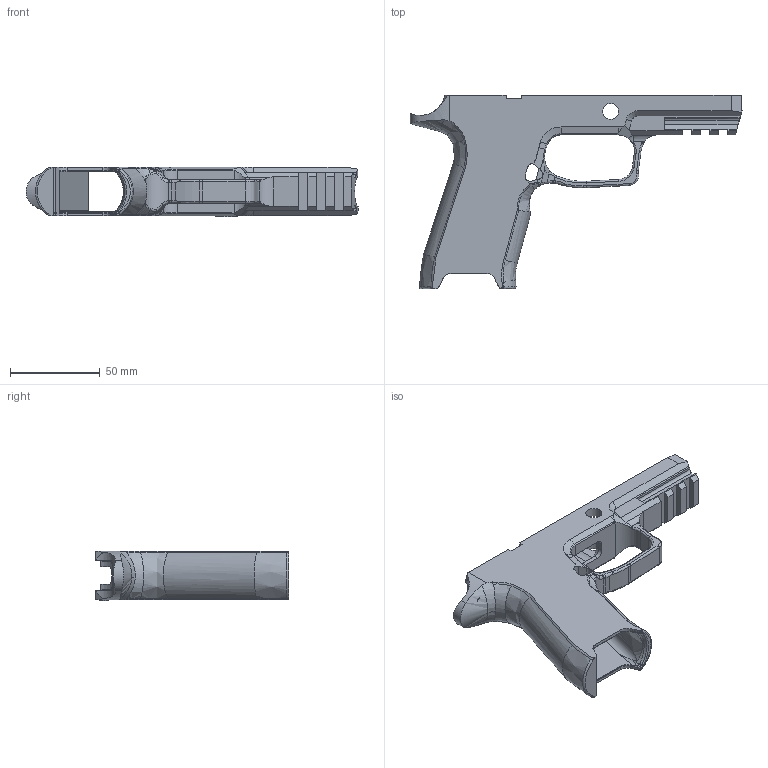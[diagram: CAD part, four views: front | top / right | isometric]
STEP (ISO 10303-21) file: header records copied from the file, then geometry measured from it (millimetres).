
FILE_DESCRIPTION(/* description */ (''),/* implementation_level */ '2;1');
FILE_NAME(/* name */ 'JP320 Grip Module Blank.step',/* time_stamp */ '2022-10-03T08:18:43-04:00',/* author */ (''),/* organization */ (''),/* preprocessor_version */ 'ST-DEVELOPER v19',/* originating_system */ 'Autodesk Translation Framework v11.7.0.108',/* authorisation */ '');
FILE_SCHEMA (('AUTOMOTIVE_DESIGN { 1 0 10303 214 3 1 1 }'));
Length unit declared in the file: millimetre
Products named in the file (3): Stippled JP320 Frame; Blank For Stippling; FCU Plug
Assembly tree (2 placements, depth 2):
  Stippled JP320 Frame
    Blank For Stippling
    FCU Plug
Bounding box: 184.6 x 107.5 x 27.5 mm (x, y, z)
Volume: 75945.4 mm3; surface area: 45541.8 mm2
Topology: 2 solids, 2 shells, 494 faces, 1403 edges, 889 vertices
Faces by surface type: plane 195, bspline 137, cylinder 120, torus 29, cone 9, sphere 4
Full cylindrical faces by diameter (mm): 8.9 x1, 9.4 x1
Entity records: 20708 total; most frequent: CARTESIAN_POINT 8499, ORIENTED_EDGE 2774, DIRECTION 2248, EDGE_CURVE 1387, VERTEX_POINT 889, AXIS2_PLACEMENT_3D 769, LINE 710, VECTOR 710
